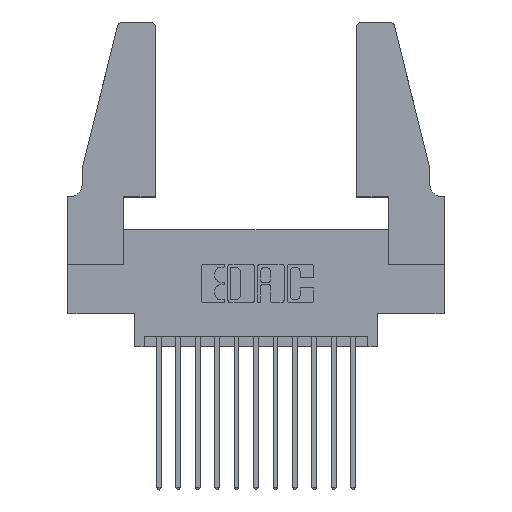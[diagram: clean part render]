
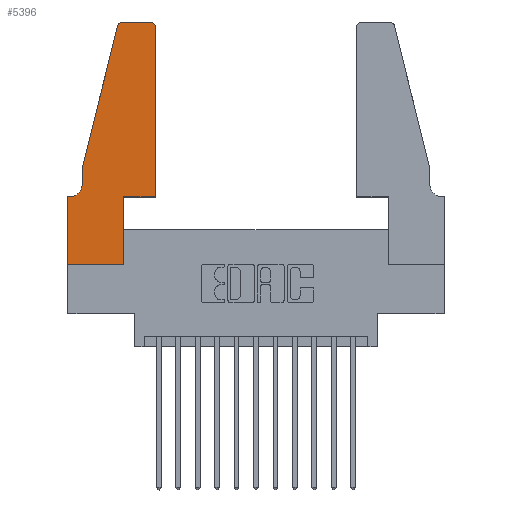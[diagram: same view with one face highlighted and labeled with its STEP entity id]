
A CAD part, top view. The second image highlights one B-rep face of the part: STEP entity #5396.
In plain terms, the highlighted planar face has unit normal (0, 0, 1).
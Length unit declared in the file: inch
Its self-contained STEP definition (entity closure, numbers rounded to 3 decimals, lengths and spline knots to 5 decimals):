
#10 = CARTESIAN_POINT ( 'NONE',  ( 0.4505, 0.35, 0.37 ) ) ;
#152 = CARTESIAN_POINT ( 'NONE',  ( 0.284, 1.22, 0.37 ) ) ;
#214 = ORIENTED_EDGE ( 'NONE', *, *, #1988, .T. ) ;
#219 = ORIENTED_EDGE ( 'NONE', *, *, #11439, .T. ) ;
#546 = VERTEX_POINT ( 'NONE', #3508 ) ;
#636 = CARTESIAN_POINT ( 'NONE',  ( 0.2865, 0., 0.37 ) ) ;
#653 = EDGE_CURVE ( 'NONE', #4489, #11466, #15036, .T. ) ;
#857 = LINE ( 'NONE', #10142, #12932 ) ;
#1546 = VERTEX_POINT ( 'NONE', #9854 ) ;
#1586 = CARTESIAN_POINT ( 'NONE',  ( 0.25487, 1.22718, 0.37 ) ) ;
#1776 = VECTOR ( 'NONE', #11975, 39.37008 ) ;
#1834 = VECTOR ( 'NONE', #4700, 39.37008 ) ;
#1838 = ORIENTED_EDGE ( 'NONE', *, *, #4472, .T. ) ;
#1853 = CARTESIAN_POINT ( 'NONE',  ( 0.4505, 1.22, 0.37 ) ) ;
#1988 = EDGE_CURVE ( 'NONE', #10748, #10691, #14992, .T. ) ;
#2010 = CARTESIAN_POINT ( 'NONE',  ( 0., 0., 0.37 ) ) ;
#2347 = CARTESIAN_POINT ( 'NONE',  ( 0.4205, 1.25, 0.37 ) ) ;
#2440 = CARTESIAN_POINT ( 'NONE',  ( 0.2865, 0.35, 0.37 ) ) ;
#2454 = AXIS2_PLACEMENT_3D ( 'NONE', #4121, #8830, #14664 ) ;
#2552 = DIRECTION ( 'NONE',  ( -1., 0., 0. ) ) ;
#2601 = CARTESIAN_POINT ( 'NONE',  ( 0.2605, 1.25, 0.37 ) ) ;
#2664 = EDGE_CURVE ( 'NONE', #11466, #4391, #4185, .T. ) ;
#2985 = EDGE_CURVE ( 'NONE', #9290, #10748, #3820, .T. ) ;
#3006 = DIRECTION ( 'NONE',  ( 0., -1., 0. ) ) ;
#3110 = CARTESIAN_POINT ( 'NONE',  ( 0.4205, 1.22, 0.37 ) ) ;
#3508 = CARTESIAN_POINT ( 'NONE',  ( 0.0755, 0.42, 0.37 ) ) ;
#3607 = DIRECTION ( 'NONE',  ( 0., 0., 1. ) ) ;
#3717 = CARTESIAN_POINT ( 'NONE',  ( 0.4505, 0.35, 0.37 ) ) ;
#3748 = FACE_OUTER_BOUND ( 'NONE', #13002, .T. ) ;
#3820 = LINE ( 'NONE', #12776, #6391 ) ;
#4121 = CARTESIAN_POINT ( 'NONE',  ( 0.0055, 0.42, 0.37 ) ) ;
#4185 = CIRCLE ( 'NONE', #13605, 0.03 ) ;
#4365 = VECTOR ( 'NONE', #13364, 39.37008 ) ;
#4391 = VERTEX_POINT ( 'NONE', #2347 ) ;
#4409 = EDGE_CURVE ( 'NONE', #10691, #1546, #9241, .T. ) ;
#4472 = EDGE_CURVE ( 'NONE', #4391, #14367, #4498, .T. ) ;
#4489 = VERTEX_POINT ( 'NONE', #3717 ) ;
#4498 = LINE ( 'NONE', #2601, #14927 ) ;
#4559 = EDGE_CURVE ( 'NONE', #14367, #11994, #5792, .T. ) ;
#4650 = CARTESIAN_POINT ( 'NONE',  ( 0.0755, 0.5, 0.37 ) ) ;
#4700 = DIRECTION ( 'NONE',  ( 1., 0., 0. ) ) ;
#4744 = EDGE_CURVE ( 'NONE', #11994, #5103, #13281, .T. ) ;
#4901 = DIRECTION ( 'NONE',  ( 0., 1., 0. ) ) ;
#5103 = VERTEX_POINT ( 'NONE', #9378 ) ;
#5108 = DIRECTION ( 'NONE',  ( 0., 0., 1. ) ) ;
#5152 = VECTOR ( 'NONE', #7158, 39.37008 ) ;
#5396 = ADVANCED_FACE ( 'NONE', ( #3748 ), #9888, .T. ) ;
#5481 = LINE ( 'NONE', #10, #1834 ) ;
#5570 = DIRECTION ( 'NONE',  ( 0., 0., 1. ) ) ;
#5668 = DIRECTION ( 'NONE',  ( 1., 0., 0. ) ) ;
#5690 = DIRECTION ( 'NONE',  ( 0., -1., 0. ) ) ;
#5792 = CIRCLE ( 'NONE', #7649, 0.03 ) ;
#5900 = CARTESIAN_POINT ( 'NONE',  ( 0., 0., 0.37 ) ) ;
#6012 = ORIENTED_EDGE ( 'NONE', *, *, #4744, .T. ) ;
#6285 = CARTESIAN_POINT ( 'NONE',  ( 0.284, 1.25, 0.37 ) ) ;
#6306 = EDGE_CURVE ( 'NONE', #1546, #4489, #5481, .T. ) ;
#6325 = CARTESIAN_POINT ( 'NONE',  ( 0.0755, 0.35, 0.37 ) ) ;
#6391 = VECTOR ( 'NONE', #5690, 39.37008 ) ;
#6447 = ORIENTED_EDGE ( 'NONE', *, *, #2985, .T. ) ;
#6637 = VECTOR ( 'NONE', #4901, 39.37008 ) ;
#6761 = AXIS2_PLACEMENT_3D ( 'NONE', #7590, #5108, #13276 ) ;
#6802 = VERTEX_POINT ( 'NONE', #14859 ) ;
#7090 = CARTESIAN_POINT ( 'NONE',  ( 0., 0.35, 0.37 ) ) ;
#7158 = DIRECTION ( 'NONE',  ( 1., 0., 0. ) ) ;
#7302 = EDGE_CURVE ( 'NONE', #5103, #546, #857, .T. ) ;
#7590 = CARTESIAN_POINT ( 'NONE',  ( 0., 0.35, 0.37 ) ) ;
#7649 = AXIS2_PLACEMENT_3D ( 'NONE', #152, #3607, #10680 ) ;
#7688 = CIRCLE ( 'NONE', #2454, 0.07 ) ;
#7691 = ORIENTED_EDGE ( 'NONE', *, *, #653, .T. ) ;
#8830 = DIRECTION ( 'NONE',  ( 0., 0., -1. ) ) ;
#9053 = VECTOR ( 'NONE', #12908, 39.37008 ) ;
#9236 = ORIENTED_EDGE ( 'NONE', *, *, #7302, .T. ) ;
#9241 = LINE ( 'NONE', #2440, #9053 ) ;
#9290 = VERTEX_POINT ( 'NONE', #7090 ) ;
#9378 = CARTESIAN_POINT ( 'NONE',  ( 0.0755, 0.5, 0.37 ) ) ;
#9854 = CARTESIAN_POINT ( 'NONE',  ( 0.2865, 0.35, 0.37 ) ) ;
#9881 = ORIENTED_EDGE ( 'NONE', *, *, #6306, .T. ) ;
#9888 = PLANE ( 'NONE',  #6761 ) ;
#10142 = CARTESIAN_POINT ( 'NONE',  ( 0.0755, 0.5, 0.37 ) ) ;
#10398 = ORIENTED_EDGE ( 'NONE', *, *, #2664, .T. ) ;
#10680 = DIRECTION ( 'NONE',  ( 1., 0., 0. ) ) ;
#10691 = VERTEX_POINT ( 'NONE', #636 ) ;
#10748 = VERTEX_POINT ( 'NONE', #2010 ) ;
#10835 = CARTESIAN_POINT ( 'NONE',  ( 0.4505, 0.35, 0.37 ) ) ;
#11413 = ORIENTED_EDGE ( 'NONE', *, *, #4409, .T. ) ;
#11439 = EDGE_CURVE ( 'NONE', #546, #6802, #7688, .T. ) ;
#11466 = VERTEX_POINT ( 'NONE', #1853 ) ;
#11500 = LINE ( 'NONE', #6325, #4365 ) ;
#11975 = DIRECTION ( 'NONE',  ( -0.239, -0.971, 0. ) ) ;
#11989 = EDGE_CURVE ( 'NONE', #6802, #9290, #11500, .T. ) ;
#11994 = VERTEX_POINT ( 'NONE', #1586 ) ;
#12063 = ORIENTED_EDGE ( 'NONE', *, *, #11989, .T. ) ;
#12776 = CARTESIAN_POINT ( 'NONE',  ( 0., 0., 0.37 ) ) ;
#12908 = DIRECTION ( 'NONE',  ( 0., 1., 0. ) ) ;
#12932 = VECTOR ( 'NONE', #3006, 39.37008 ) ;
#13002 = EDGE_LOOP ( 'NONE', ( #1838, #13123, #6012, #9236, #219, #12063, #6447, #214, #11413, #9881, #7691, #10398 ) ) ;
#13123 = ORIENTED_EDGE ( 'NONE', *, *, #4559, .T. ) ;
#13276 = DIRECTION ( 'NONE',  ( 1., 0., 0. ) ) ;
#13281 = LINE ( 'NONE', #4650, #1776 ) ;
#13364 = DIRECTION ( 'NONE',  ( -1., 0., 0. ) ) ;
#13605 = AXIS2_PLACEMENT_3D ( 'NONE', #3110, #5570, #5668 ) ;
#14367 = VERTEX_POINT ( 'NONE', #6285 ) ;
#14664 = DIRECTION ( 'NONE',  ( -1., 0., 0. ) ) ;
#14859 = CARTESIAN_POINT ( 'NONE',  ( 0.0055, 0.35, 0.37 ) ) ;
#14927 = VECTOR ( 'NONE', #2552, 39.37008 ) ;
#14992 = LINE ( 'NONE', #5900, #5152 ) ;
#15036 = LINE ( 'NONE', #10835, #6637 ) ;
